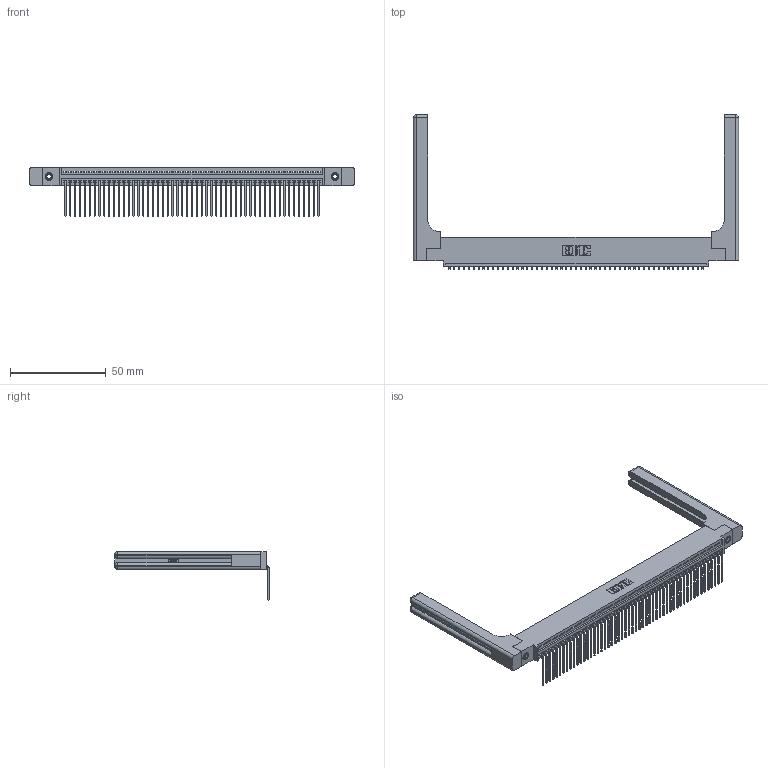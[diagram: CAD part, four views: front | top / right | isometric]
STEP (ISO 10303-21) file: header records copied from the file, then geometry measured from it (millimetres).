
FILE_DESCRIPTION (( 'STEP AP203' ), '1' );
FILE_NAME ('345-053-559-458.STEP', '2019-10-09T22:12:43', ( '' ), ( '' ), 'SwSTEP 2.0', 'SolidWorks 2016', '' );
FILE_SCHEMA (( 'CONFIG_CONTROL_DESIGN' ));
Length unit declared in the file: inch
Products named in the file (5): 345-220-058_345-220-058; 345 Part_0.110 Offset - 0.156 Dia-TH; 345-053-559-458; 345-292-001_558 559 Tail - 1; 345-250-001_345-250-001-102
Assembly tree (58 placements, depth 2):
  345-053-559-458
    345 Part_0.110 Offset - 0.156 Dia-TH
    345-292-001_558 559 Tail - 1  x53
    345-250-001_345-250-001-102  x2
    345-220-058_345-220-058  x2
Bounding box: 169.65 x 80.51 x 25.53 mm (x, y, z)
Volume: 24811.5 mm3; surface area: 28244.5 mm2
Topology: 58 solids, 58 shells, 3566 faces, 10665 edges, 7018 vertices
Faces by surface type: plane 2458, cylinder 1048, bspline 36, cone 12, sphere 8, torus 4
Entity records: 43806 total; most frequent: CARTESIAN_POINT 8560, ORIENTED_EDGE 7344, DIRECTION 6406, EDGE_CURVE 3672, VECTOR 3236, LINE 3236, VERTEX_POINT 2438, AXIS2_PLACEMENT_3D 1585
